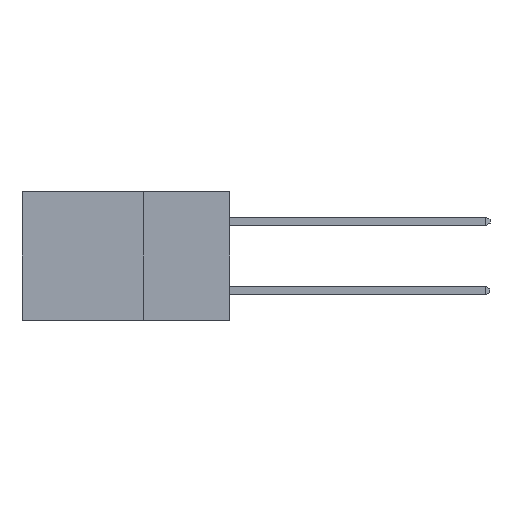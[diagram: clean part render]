
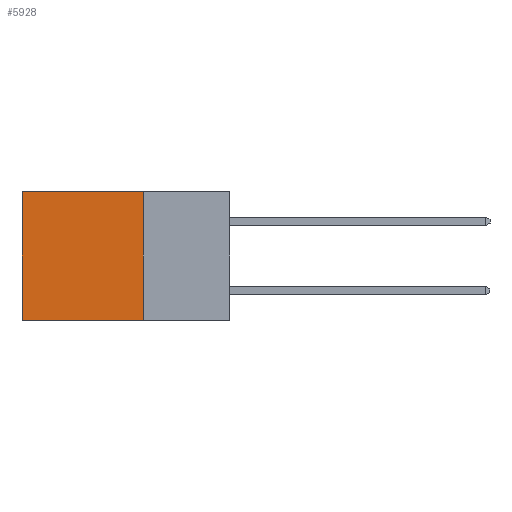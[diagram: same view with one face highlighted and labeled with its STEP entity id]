
A CAD part, left-side view. The second image highlights one B-rep face of the part: STEP entity #5928.
In plain terms, the highlighted planar face has unit normal (-1, 0, 0).
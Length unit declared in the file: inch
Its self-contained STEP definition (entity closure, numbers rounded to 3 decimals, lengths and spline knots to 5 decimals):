
#583 = VERTEX_POINT ( 'NONE', #3686 ) ;
#1434 = CARTESIAN_POINT ( 'NONE',  ( 0.298, 0.25, 0. ) ) ;
#1979 = EDGE_CURVE ( 'NONE', #11493, #14369, #7093, .T. ) ;
#2450 = VERTEX_POINT ( 'NONE', #8493 ) ;
#3686 = CARTESIAN_POINT ( 'NONE',  ( 0.298, 0.6, -0.37 ) ) ;
#4654 = CARTESIAN_POINT ( 'NONE',  ( 0.298, 0.6, 0. ) ) ;
#4660 = EDGE_CURVE ( 'NONE', #11493, #2450, #5083, .T. ) ;
#5083 = LINE ( 'NONE', #10531, #7715 ) ;
#5834 = VECTOR ( 'NONE', #13807, 39.37008 ) ;
#5865 = CARTESIAN_POINT ( 'NONE',  ( 0.298, 0.6, 0. ) ) ;
#5928 = ADVANCED_FACE ( 'NONE', ( #13679 ), #9349, .F. ) ;
#6285 = VECTOR ( 'NONE', #10614, 39.37008 ) ;
#6909 = EDGE_CURVE ( 'NONE', #14369, #583, #12269, .T. ) ;
#7093 = LINE ( 'NONE', #1434, #9387 ) ;
#7492 = EDGE_LOOP ( 'NONE', ( #12689, #12356, #7735, #14436 ) ) ;
#7715 = VECTOR ( 'NONE', #11319, 39.37008 ) ;
#7735 = ORIENTED_EDGE ( 'NONE', *, *, #4660, .F. ) ;
#8139 = CARTESIAN_POINT ( 'NONE',  ( 0.298, 0.25, 0. ) ) ;
#8493 = CARTESIAN_POINT ( 'NONE',  ( 0.298, 0.25, -0.37 ) ) ;
#8925 = DIRECTION ( 'NONE',  ( 0., 0., -1. ) ) ;
#9041 = DIRECTION ( 'NONE',  ( 1., 0., 0. ) ) ;
#9317 = CARTESIAN_POINT ( 'NONE',  ( 0.298, 0.25, 0. ) ) ;
#9349 = PLANE ( 'NONE',  #12443 ) ;
#9387 = VECTOR ( 'NONE', #14428, 39.37008 ) ;
#10531 = CARTESIAN_POINT ( 'NONE',  ( 0.298, 0.25, 0. ) ) ;
#10614 = DIRECTION ( 'NONE',  ( 0., 0., -1. ) ) ;
#10652 = EDGE_CURVE ( 'NONE', #2450, #583, #11815, .T. ) ;
#11319 = DIRECTION ( 'NONE',  ( 0., 0., -1. ) ) ;
#11493 = VERTEX_POINT ( 'NONE', #8139 ) ;
#11815 = LINE ( 'NONE', #13935, #5834 ) ;
#12269 = LINE ( 'NONE', #5865, #6285 ) ;
#12356 = ORIENTED_EDGE ( 'NONE', *, *, #10652, .F. ) ;
#12443 = AXIS2_PLACEMENT_3D ( 'NONE', #9317, #9041, #8925 ) ;
#12689 = ORIENTED_EDGE ( 'NONE', *, *, #6909, .T. ) ;
#13679 = FACE_OUTER_BOUND ( 'NONE', #7492, .T. ) ;
#13807 = DIRECTION ( 'NONE',  ( 0., 1., 0. ) ) ;
#13935 = CARTESIAN_POINT ( 'NONE',  ( 0.298, 0.25, -0.37 ) ) ;
#14369 = VERTEX_POINT ( 'NONE', #4654 ) ;
#14428 = DIRECTION ( 'NONE',  ( 0., 1., 0. ) ) ;
#14436 = ORIENTED_EDGE ( 'NONE', *, *, #1979, .T. ) ;
